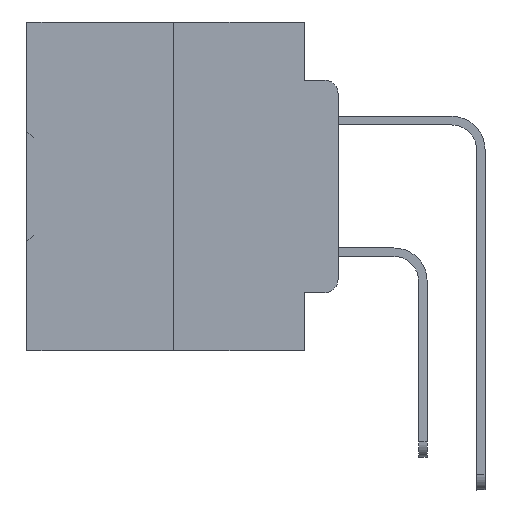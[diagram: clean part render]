
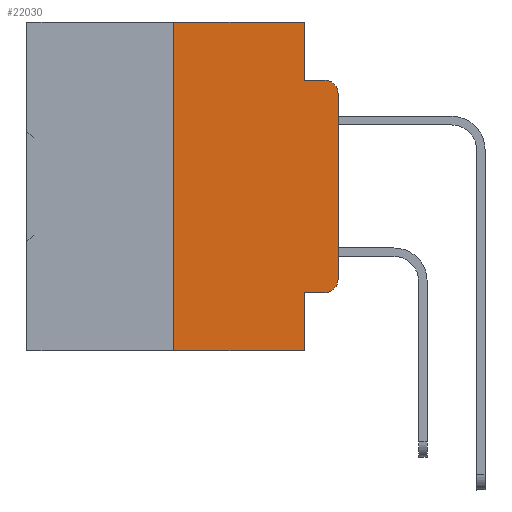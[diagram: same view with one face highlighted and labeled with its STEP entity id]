
A CAD part, left-side view. The second image highlights one B-rep face of the part: STEP entity #22030.
In plain terms, the highlighted planar face has unit normal (-1, 0, 0).
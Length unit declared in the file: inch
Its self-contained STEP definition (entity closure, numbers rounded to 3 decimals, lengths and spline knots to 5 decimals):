
#89 = FACE_OUTER_BOUND ( 'NONE', #32684, .T. ) ;
#493 = DIRECTION ( 'NONE',  ( 0., 0., -1. ) ) ;
#639 = CARTESIAN_POINT ( 'NONE',  ( 0., 0.25, 0. ) ) ;
#1250 = CARTESIAN_POINT ( 'NONE',  ( 0., 0.051, 0. ) ) ;
#1324 = ORIENTED_EDGE ( 'NONE', *, *, #4422, .F. ) ;
#2431 = LINE ( 'NONE', #23671, #33125 ) ;
#2461 = ORIENTED_EDGE ( 'NONE', *, *, #25488, .T. ) ;
#2539 = DIRECTION ( 'NONE',  ( -1., 0., 0. ) ) ;
#2736 = CARTESIAN_POINT ( 'NONE',  ( 0., 0.02, -0.1085 ) ) ;
#3128 = CARTESIAN_POINT ( 'NONE',  ( 0., 0., 0. ) ) ;
#3305 = LINE ( 'NONE', #9517, #9653 ) ;
#3315 = EDGE_CURVE ( 'NONE', #22212, #13676, #17288, .T. ) ;
#3908 = VECTOR ( 'NONE', #29629, 39.37008 ) ;
#4422 = EDGE_CURVE ( 'NONE', #22081, #17074, #18224, .T. ) ;
#5146 = LINE ( 'NONE', #20551, #9755 ) ;
#5866 = ORIENTED_EDGE ( 'NONE', *, *, #3315, .T. ) ;
#6360 = CARTESIAN_POINT ( 'NONE',  ( 0., 0.051, -0.5 ) ) ;
#7689 = DIRECTION ( 'NONE',  ( 0., -1., 0. ) ) ;
#7765 = AXIS2_PLACEMENT_3D ( 'NONE', #2736, #2539, #32583 ) ;
#8891 = VERTEX_POINT ( 'NONE', #15525 ) ;
#8938 = PLANE ( 'NONE',  #28022 ) ;
#9003 = CARTESIAN_POINT ( 'NONE',  ( 0., 0.473, 0. ) ) ;
#9125 = DIRECTION ( 'NONE',  ( 0., -1., 0. ) ) ;
#9517 = CARTESIAN_POINT ( 'NONE',  ( 0., 0.051, -0.0885 ) ) ;
#9653 = VECTOR ( 'NONE', #9125, 39.37008 ) ;
#9755 = VECTOR ( 'NONE', #21142, 39.37008 ) ;
#9954 = VECTOR ( 'NONE', #7689, 39.37008 ) ;
#10339 = ORIENTED_EDGE ( 'NONE', *, *, #26856, .F. ) ;
#10666 = AXIS2_PLACEMENT_3D ( 'NONE', #37680, #18654, #13052 ) ;
#10926 = ORIENTED_EDGE ( 'NONE', *, *, #32269, .F. ) ;
#11002 = EDGE_CURVE ( 'NONE', #25756, #8891, #20883, .T. ) ;
#11779 = ORIENTED_EDGE ( 'NONE', *, *, #17336, .F. ) ;
#11803 = VECTOR ( 'NONE', #30827, 39.37008 ) ;
#12016 = LINE ( 'NONE', #9003, #3908 ) ;
#12227 = CARTESIAN_POINT ( 'NONE',  ( 0., 0.051, 0. ) ) ;
#13052 = DIRECTION ( 'NONE',  ( 0., 0., -1. ) ) ;
#13676 = VERTEX_POINT ( 'NONE', #6360 ) ;
#13925 = CARTESIAN_POINT ( 'NONE',  ( 0., 0.02, -0.4115 ) ) ;
#14078 = LINE ( 'NONE', #1250, #32026 ) ;
#14360 = ORIENTED_EDGE ( 'NONE', *, *, #37601, .T. ) ;
#15134 = ORIENTED_EDGE ( 'NONE', *, *, #35706, .F. ) ;
#15333 = DIRECTION ( 'NONE',  ( 0., 0., 1. ) ) ;
#15525 = CARTESIAN_POINT ( 'NONE',  ( 0., 0., -0.3915 ) ) ;
#15717 = CARTESIAN_POINT ( 'NONE',  ( 0., 0.473, 0. ) ) ;
#15746 = CARTESIAN_POINT ( 'NONE',  ( 0., 0., -0.1085 ) ) ;
#17074 = VERTEX_POINT ( 'NONE', #27512 ) ;
#17288 = LINE ( 'NONE', #29502, #9954 ) ;
#17336 = EDGE_CURVE ( 'NONE', #19386, #13676, #14078, .T. ) ;
#17350 = VERTEX_POINT ( 'NONE', #31902 ) ;
#18224 = LINE ( 'NONE', #12227, #11803 ) ;
#18344 = LINE ( 'NONE', #3128, #33853 ) ;
#18523 = VERTEX_POINT ( 'NONE', #15746 ) ;
#18654 = DIRECTION ( 'NONE',  ( -1., 0., 0. ) ) ;
#19386 = VERTEX_POINT ( 'NONE', #27610 ) ;
#19910 = CIRCLE ( 'NONE', #7765, 0.02 ) ;
#20551 = CARTESIAN_POINT ( 'NONE',  ( 0., 0.051, -0.4115 ) ) ;
#20883 = CIRCLE ( 'NONE', #10666, 0.02 ) ;
#20936 = CARTESIAN_POINT ( 'NONE',  ( 0., 0.051, 0. ) ) ;
#21142 = DIRECTION ( 'NONE',  ( 0., -1., 0. ) ) ;
#22030 = ADVANCED_FACE ( 'NONE', ( #89 ), #8938, .F. ) ;
#22081 = VERTEX_POINT ( 'NONE', #20936 ) ;
#22212 = VERTEX_POINT ( 'NONE', #28325 ) ;
#23671 = CARTESIAN_POINT ( 'NONE',  ( 0., 0.25, 0. ) ) ;
#24146 = ORIENTED_EDGE ( 'NONE', *, *, #11002, .T. ) ;
#25488 = EDGE_CURVE ( 'NONE', #8891, #18523, #18344, .T. ) ;
#25756 = VERTEX_POINT ( 'NONE', #13925 ) ;
#26856 = EDGE_CURVE ( 'NONE', #36220, #22081, #12016, .T. ) ;
#26866 = DIRECTION ( 'NONE',  ( 0., 0., 1. ) ) ;
#27512 = CARTESIAN_POINT ( 'NONE',  ( 0., 0.051, -0.0885 ) ) ;
#27610 = CARTESIAN_POINT ( 'NONE',  ( 0., 0.051, -0.4115 ) ) ;
#27928 = DIRECTION ( 'NONE',  ( 1., 0., 0. ) ) ;
#28022 = AXIS2_PLACEMENT_3D ( 'NONE', #15717, #27928, #493 ) ;
#28325 = CARTESIAN_POINT ( 'NONE',  ( 0., 0.25, -0.5 ) ) ;
#29502 = CARTESIAN_POINT ( 'NONE',  ( 0., 0.473, -0.5 ) ) ;
#29555 = ORIENTED_EDGE ( 'NONE', *, *, #29928, .T. ) ;
#29629 = DIRECTION ( 'NONE',  ( 0., -1., 0. ) ) ;
#29928 = EDGE_CURVE ( 'NONE', #19386, #25756, #5146, .T. ) ;
#30827 = DIRECTION ( 'NONE',  ( 0., 0., -1. ) ) ;
#31902 = CARTESIAN_POINT ( 'NONE',  ( 0., 0.02, -0.0885 ) ) ;
#32026 = VECTOR ( 'NONE', #37912, 39.37008 ) ;
#32269 = EDGE_CURVE ( 'NONE', #22212, #36220, #2431, .T. ) ;
#32583 = DIRECTION ( 'NONE',  ( 0., 0., -1. ) ) ;
#32684 = EDGE_LOOP ( 'NONE', ( #2461, #14360, #15134, #1324, #10339, #10926, #5866, #11779, #29555, #24146 ) ) ;
#33125 = VECTOR ( 'NONE', #26866, 39.37008 ) ;
#33853 = VECTOR ( 'NONE', #15333, 39.37008 ) ;
#35706 = EDGE_CURVE ( 'NONE', #17074, #17350, #3305, .T. ) ;
#36220 = VERTEX_POINT ( 'NONE', #639 ) ;
#37601 = EDGE_CURVE ( 'NONE', #18523, #17350, #19910, .T. ) ;
#37680 = CARTESIAN_POINT ( 'NONE',  ( 0., 0.02, -0.3915 ) ) ;
#37912 = DIRECTION ( 'NONE',  ( 0., 0., -1. ) ) ;
